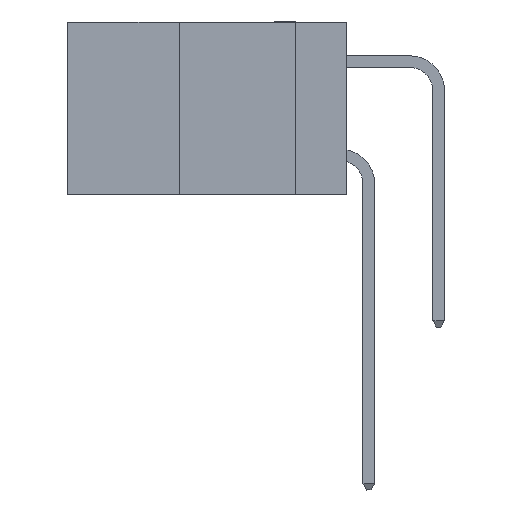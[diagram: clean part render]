
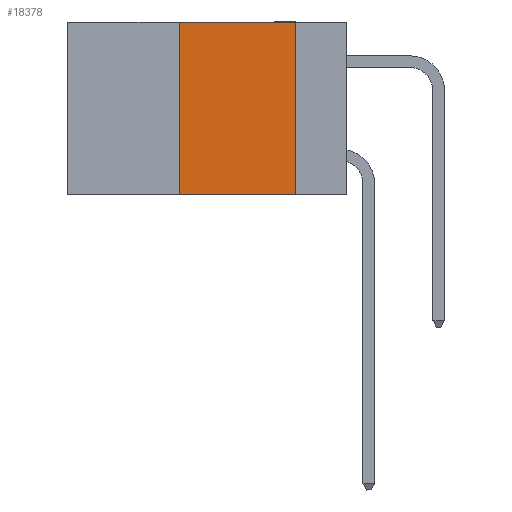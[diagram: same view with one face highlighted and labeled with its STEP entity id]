
A CAD part, left-side view. The second image highlights one B-rep face of the part: STEP entity #18378.
In plain terms, the highlighted planar face has unit normal (-1, 0, 0).
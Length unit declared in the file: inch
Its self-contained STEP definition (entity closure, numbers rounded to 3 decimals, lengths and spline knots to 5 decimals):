
#402 = DIRECTION ( 'NONE',  ( 0., -1., 0. ) ) ;
#545 = CARTESIAN_POINT ( 'NONE',  ( 0., 0.11, -0.37 ) ) ;
#2160 = AXIS2_PLACEMENT_3D ( 'NONE', #14964, #18033, #7436 ) ;
#2740 = ORIENTED_EDGE ( 'NONE', *, *, #8410, .F. ) ;
#3733 = VECTOR ( 'NONE', #16015, 39.37008 ) ;
#4455 = PLANE ( 'NONE',  #2160 ) ;
#4470 = VERTEX_POINT ( 'NONE', #545 ) ;
#5077 = VECTOR ( 'NONE', #19120, 39.37008 ) ;
#5514 = CARTESIAN_POINT ( 'NONE',  ( 0., 0.11, 0. ) ) ;
#6223 = FACE_OUTER_BOUND ( 'NONE', #8435, .T. ) ;
#6696 = CARTESIAN_POINT ( 'NONE',  ( 0., 0.6, 0. ) ) ;
#7436 = DIRECTION ( 'NONE',  ( 0., 0., -1. ) ) ;
#7772 = LINE ( 'NONE', #5514, #3733 ) ;
#8334 = EDGE_CURVE ( 'NONE', #18654, #18353, #8879, .T. ) ;
#8410 = EDGE_CURVE ( 'NONE', #18450, #18654, #11950, .T. ) ;
#8435 = EDGE_LOOP ( 'NONE', ( #16075, #11599, #2740, #8552 ) ) ;
#8476 = CARTESIAN_POINT ( 'NONE',  ( 0., 0.36, 0. ) ) ;
#8552 = ORIENTED_EDGE ( 'NONE', *, *, #17594, .T. ) ;
#8879 = LINE ( 'NONE', #6696, #12654 ) ;
#9284 = CARTESIAN_POINT ( 'NONE',  ( 0., 0.36, -0.37 ) ) ;
#9484 = CARTESIAN_POINT ( 'NONE',  ( 0., 0.36, 0. ) ) ;
#10279 = LINE ( 'NONE', #17990, #17921 ) ;
#11599 = ORIENTED_EDGE ( 'NONE', *, *, #8334, .F. ) ;
#11950 = LINE ( 'NONE', #8476, #5077 ) ;
#12654 = VECTOR ( 'NONE', #402, 39.37008 ) ;
#14781 = EDGE_CURVE ( 'NONE', #18353, #4470, #7772, .T. ) ;
#14964 = CARTESIAN_POINT ( 'NONE',  ( 0., 0.6, 0. ) ) ;
#16015 = DIRECTION ( 'NONE',  ( 0., 0., -1. ) ) ;
#16075 = ORIENTED_EDGE ( 'NONE', *, *, #14781, .F. ) ;
#16561 = CARTESIAN_POINT ( 'NONE',  ( 0., 0.11, 0. ) ) ;
#17594 = EDGE_CURVE ( 'NONE', #18450, #4470, #10279, .T. ) ;
#17921 = VECTOR ( 'NONE', #19309, 39.37008 ) ;
#17990 = CARTESIAN_POINT ( 'NONE',  ( 0., 0.6, -0.37 ) ) ;
#18033 = DIRECTION ( 'NONE',  ( 1., 0., 0. ) ) ;
#18353 = VERTEX_POINT ( 'NONE', #16561 ) ;
#18378 = ADVANCED_FACE ( 'NONE', ( #6223 ), #4455, .F. ) ;
#18450 = VERTEX_POINT ( 'NONE', #9284 ) ;
#18654 = VERTEX_POINT ( 'NONE', #9484 ) ;
#19120 = DIRECTION ( 'NONE',  ( 0., 0., 1. ) ) ;
#19309 = DIRECTION ( 'NONE',  ( 0., -1., 0. ) ) ;
